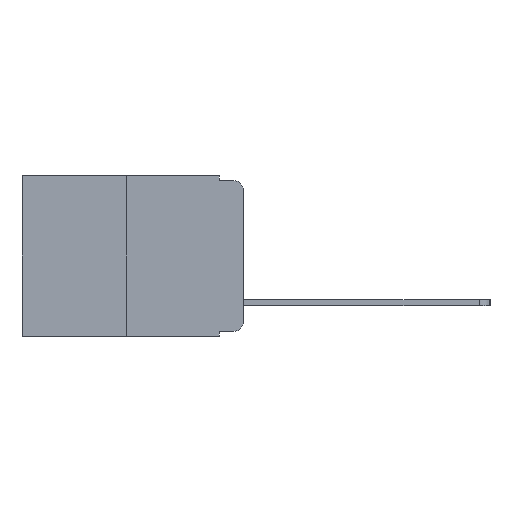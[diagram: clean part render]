
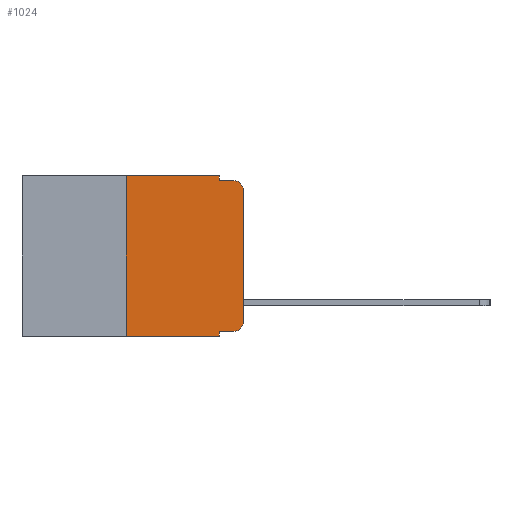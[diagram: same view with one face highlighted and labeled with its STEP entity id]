
A CAD part, left-side view. The second image highlights one B-rep face of the part: STEP entity #1024.
In plain terms, the highlighted planar face has unit normal (-1, 0, 0).
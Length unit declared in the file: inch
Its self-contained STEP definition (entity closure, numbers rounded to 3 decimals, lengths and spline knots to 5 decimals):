
#5 = ORIENTED_EDGE ( 'NONE', *, *, #8488, .T. ) ;
#14 = ORIENTED_EDGE ( 'NONE', *, *, #4066, .F. ) ;
#179 = VERTEX_POINT ( 'NONE', #1207 ) ;
#283 = EDGE_LOOP ( 'NONE', ( #10477, #7204, #2831, #1139, #8555, #8171, #9225, #14, #5, #5993 ) ) ;
#448 = VERTEX_POINT ( 'NONE', #10033 ) ;
#524 = VECTOR ( 'NONE', #4767, 39.37008 ) ;
#657 = VERTEX_POINT ( 'NONE', #4558 ) ;
#737 = CARTESIAN_POINT ( 'NONE',  ( 0., 0.051, 0. ) ) ;
#771 = VERTEX_POINT ( 'NONE', #9033 ) ;
#915 = VERTEX_POINT ( 'NONE', #10164 ) ;
#994 = DIRECTION ( 'NONE',  ( 0., -1., 0. ) ) ;
#1024 = ADVANCED_FACE ( 'NONE', ( #9141 ), #1451, .F. ) ;
#1139 = ORIENTED_EDGE ( 'NONE', *, *, #10688, .F. ) ;
#1207 = CARTESIAN_POINT ( 'NONE',  ( 0., 0.051, 0. ) ) ;
#1451 = PLANE ( 'NONE',  #9640 ) ;
#1633 = CARTESIAN_POINT ( 'NONE',  ( 0., 0.25, 0. ) ) ;
#1849 = EDGE_CURVE ( 'NONE', #7799, #179, #4304, .T. ) ;
#1965 = VECTOR ( 'NONE', #8818, 39.37008 ) ;
#2428 = EDGE_CURVE ( 'NONE', #3110, #657, #3740, .T. ) ;
#2600 = DIRECTION ( 'NONE',  ( -1., 0., 0. ) ) ;
#2757 = VECTOR ( 'NONE', #7227, 39.37008 ) ;
#2781 = CARTESIAN_POINT ( 'NONE',  ( 0., 0.02, -0.03 ) ) ;
#2831 = ORIENTED_EDGE ( 'NONE', *, *, #8124, .F. ) ;
#2877 = LINE ( 'NONE', #4985, #4902 ) ;
#3049 = CARTESIAN_POINT ( 'NONE',  ( 0., 0.25, 0. ) ) ;
#3110 = VERTEX_POINT ( 'NONE', #9869 ) ;
#3122 = AXIS2_PLACEMENT_3D ( 'NONE', #2781, #2600, #8522 ) ;
#3156 = VERTEX_POINT ( 'NONE', #4901 ) ;
#3192 = VECTOR ( 'NONE', #994, 39.37008 ) ;
#3378 = CARTESIAN_POINT ( 'NONE',  ( 0., 0., -0.313 ) ) ;
#3525 = VERTEX_POINT ( 'NONE', #3378 ) ;
#3740 = LINE ( 'NONE', #6244, #3192 ) ;
#3823 = VECTOR ( 'NONE', #6267, 39.37008 ) ;
#3953 = AXIS2_PLACEMENT_3D ( 'NONE', #9959, #5176, #10689 ) ;
#4066 = EDGE_CURVE ( 'NONE', #915, #657, #9095, .T. ) ;
#4254 = CARTESIAN_POINT ( 'NONE',  ( 0., 0.473, 0. ) ) ;
#4304 = LINE ( 'NONE', #10571, #1965 ) ;
#4461 = VECTOR ( 'NONE', #6216, 39.37008 ) ;
#4558 = CARTESIAN_POINT ( 'NONE',  ( 0., 0.051, -0.343 ) ) ;
#4719 = LINE ( 'NONE', #8655, #4461 ) ;
#4767 = DIRECTION ( 'NONE',  ( 0., 0., 1. ) ) ;
#4850 = DIRECTION ( 'NONE',  ( 1., 0., 0. ) ) ;
#4860 = EDGE_CURVE ( 'NONE', #3525, #3156, #8188, .T. ) ;
#4901 = CARTESIAN_POINT ( 'NONE',  ( 0., 0., -0.03 ) ) ;
#4902 = VECTOR ( 'NONE', #5825, 39.37008 ) ;
#4985 = CARTESIAN_POINT ( 'NONE',  ( 0., 0.051, -0.333 ) ) ;
#5176 = DIRECTION ( 'NONE',  ( -1., 0., 0. ) ) ;
#5402 = DIRECTION ( 'NONE',  ( 0., -1., 0. ) ) ;
#5766 = EDGE_CURVE ( 'NONE', #3110, #7799, #9547, .T. ) ;
#5825 = DIRECTION ( 'NONE',  ( 0., -1., 0. ) ) ;
#5931 = VECTOR ( 'NONE', #5402, 39.37008 ) ;
#5993 = ORIENTED_EDGE ( 'NONE', *, *, #10521, .T. ) ;
#6216 = DIRECTION ( 'NONE',  ( 0., 0., -1. ) ) ;
#6244 = CARTESIAN_POINT ( 'NONE',  ( 0., 0.473, -0.343 ) ) ;
#6267 = DIRECTION ( 'NONE',  ( 0., 0., 1. ) ) ;
#6517 = EDGE_CURVE ( 'NONE', #3156, #771, #10628, .T. ) ;
#7204 = ORIENTED_EDGE ( 'NONE', *, *, #6517, .T. ) ;
#7227 = DIRECTION ( 'NONE',  ( 0., 0., -1. ) ) ;
#7722 = DIRECTION ( 'NONE',  ( 0., 0., -1. ) ) ;
#7799 = VERTEX_POINT ( 'NONE', #3049 ) ;
#8124 = EDGE_CURVE ( 'NONE', #448, #771, #8331, .T. ) ;
#8171 = ORIENTED_EDGE ( 'NONE', *, *, #5766, .F. ) ;
#8188 = LINE ( 'NONE', #9453, #3823 ) ;
#8331 = LINE ( 'NONE', #8633, #5931 ) ;
#8488 = EDGE_CURVE ( 'NONE', #915, #9691, #2877, .T. ) ;
#8522 = DIRECTION ( 'NONE',  ( 0., 0., -1. ) ) ;
#8555 = ORIENTED_EDGE ( 'NONE', *, *, #1849, .F. ) ;
#8633 = CARTESIAN_POINT ( 'NONE',  ( 0., 0.051, -0.01 ) ) ;
#8655 = CARTESIAN_POINT ( 'NONE',  ( 0., 0.051, 0. ) ) ;
#8818 = DIRECTION ( 'NONE',  ( 0., -1., 0. ) ) ;
#9033 = CARTESIAN_POINT ( 'NONE',  ( 0., 0.02, -0.01 ) ) ;
#9095 = LINE ( 'NONE', #737, #2757 ) ;
#9141 = FACE_OUTER_BOUND ( 'NONE', #283, .T. ) ;
#9225 = ORIENTED_EDGE ( 'NONE', *, *, #2428, .T. ) ;
#9453 = CARTESIAN_POINT ( 'NONE',  ( 0., 0., 0. ) ) ;
#9547 = LINE ( 'NONE', #1633, #524 ) ;
#9640 = AXIS2_PLACEMENT_3D ( 'NONE', #4254, #4850, #7722 ) ;
#9649 = CARTESIAN_POINT ( 'NONE',  ( 0., 0.02, -0.333 ) ) ;
#9691 = VERTEX_POINT ( 'NONE', #9649 ) ;
#9869 = CARTESIAN_POINT ( 'NONE',  ( 0., 0.25, -0.343 ) ) ;
#9959 = CARTESIAN_POINT ( 'NONE',  ( 0., 0.02, -0.313 ) ) ;
#10033 = CARTESIAN_POINT ( 'NONE',  ( 0., 0.051, -0.01 ) ) ;
#10164 = CARTESIAN_POINT ( 'NONE',  ( 0., 0.051, -0.333 ) ) ;
#10213 = CIRCLE ( 'NONE', #3953, 0.02 ) ;
#10477 = ORIENTED_EDGE ( 'NONE', *, *, #4860, .T. ) ;
#10521 = EDGE_CURVE ( 'NONE', #9691, #3525, #10213, .T. ) ;
#10571 = CARTESIAN_POINT ( 'NONE',  ( 0., 0.473, 0. ) ) ;
#10628 = CIRCLE ( 'NONE', #3122, 0.02 ) ;
#10688 = EDGE_CURVE ( 'NONE', #179, #448, #4719, .T. ) ;
#10689 = DIRECTION ( 'NONE',  ( 0., 0., -1. ) ) ;
